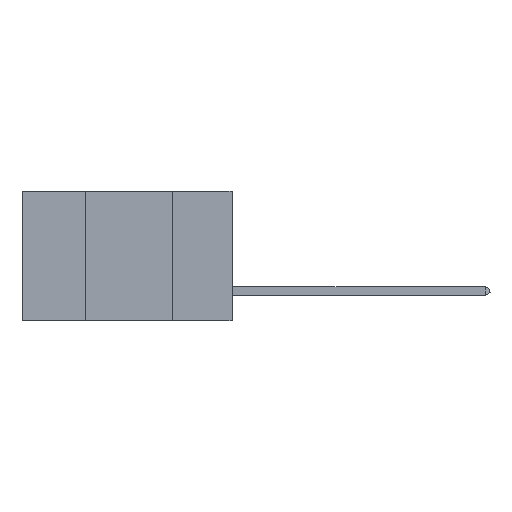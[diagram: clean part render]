
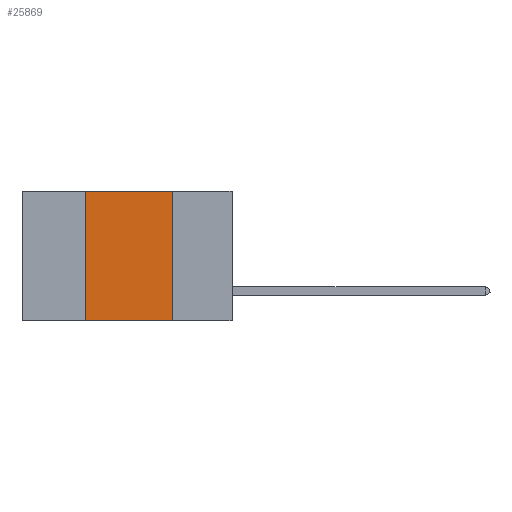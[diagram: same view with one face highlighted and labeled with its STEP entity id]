
A CAD part, left-side view. The second image highlights one B-rep face of the part: STEP entity #25869.
In plain terms, the highlighted planar face has unit normal (-1, 0, 0).
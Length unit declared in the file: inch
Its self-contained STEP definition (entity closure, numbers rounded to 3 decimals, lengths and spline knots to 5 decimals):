
#1170 = VERTEX_POINT ( 'NONE', #11110 ) ;
#1715 = ORIENTED_EDGE ( 'NONE', *, *, #15404, .F. ) ;
#2242 = EDGE_LOOP ( 'NONE', ( #1715, #49154, #13611, #39178 ) ) ;
#2798 = CARTESIAN_POINT ( 'NONE',  ( 0., 0.6, -0.37 ) ) ;
#6573 = DIRECTION ( 'NONE',  ( 0., -1., 0. ) ) ;
#10797 = DIRECTION ( 'NONE',  ( 0., -1., 0. ) ) ;
#10852 = EDGE_CURVE ( 'NONE', #1170, #24438, #24314, .T. ) ;
#11110 = CARTESIAN_POINT ( 'NONE',  ( 0., 0.42, -0.37 ) ) ;
#13611 = ORIENTED_EDGE ( 'NONE', *, *, #22544, .F. ) ;
#14380 = CARTESIAN_POINT ( 'NONE',  ( 0., 0.6, 0. ) ) ;
#14959 = CARTESIAN_POINT ( 'NONE',  ( 0., 0.17, 0. ) ) ;
#15404 = EDGE_CURVE ( 'NONE', #35234, #24438, #23323, .T. ) ;
#15495 = DIRECTION ( 'NONE',  ( 0., 0., -1. ) ) ;
#17534 = LINE ( 'NONE', #34052, #30196 ) ;
#22544 = EDGE_CURVE ( 'NONE', #1170, #26125, #17534, .T. ) ;
#23323 = LINE ( 'NONE', #38631, #26320 ) ;
#23875 = DIRECTION ( 'NONE',  ( 0., 0., -1. ) ) ;
#24314 = LINE ( 'NONE', #2798, #29174 ) ;
#24438 = VERTEX_POINT ( 'NONE', #29148 ) ;
#25869 = ADVANCED_FACE ( 'NONE', ( #37922 ), #46956, .F. ) ;
#26125 = VERTEX_POINT ( 'NONE', #40899 ) ;
#26320 = VECTOR ( 'NONE', #15495, 39.37008 ) ;
#26351 = EDGE_CURVE ( 'NONE', #26125, #35234, #47443, .T. ) ;
#27776 = CARTESIAN_POINT ( 'NONE',  ( 0., 0.6, 0. ) ) ;
#28110 = DIRECTION ( 'NONE',  ( 1., 0., 0. ) ) ;
#29148 = CARTESIAN_POINT ( 'NONE',  ( 0., 0.17, -0.37 ) ) ;
#29174 = VECTOR ( 'NONE', #10797, 39.37008 ) ;
#30196 = VECTOR ( 'NONE', #41968, 39.37008 ) ;
#34052 = CARTESIAN_POINT ( 'NONE',  ( 0., 0.42, 0. ) ) ;
#35234 = VERTEX_POINT ( 'NONE', #14959 ) ;
#37204 = VECTOR ( 'NONE', #6573, 39.37008 ) ;
#37922 = FACE_OUTER_BOUND ( 'NONE', #2242, .T. ) ;
#38631 = CARTESIAN_POINT ( 'NONE',  ( 0., 0.17, 0. ) ) ;
#39178 = ORIENTED_EDGE ( 'NONE', *, *, #10852, .T. ) ;
#40899 = CARTESIAN_POINT ( 'NONE',  ( 0., 0.42, 0. ) ) ;
#41968 = DIRECTION ( 'NONE',  ( 0., 0., 1. ) ) ;
#46956 = PLANE ( 'NONE',  #48617 ) ;
#47443 = LINE ( 'NONE', #14380, #37204 ) ;
#48617 = AXIS2_PLACEMENT_3D ( 'NONE', #27776, #28110, #23875 ) ;
#49154 = ORIENTED_EDGE ( 'NONE', *, *, #26351, .F. ) ;
